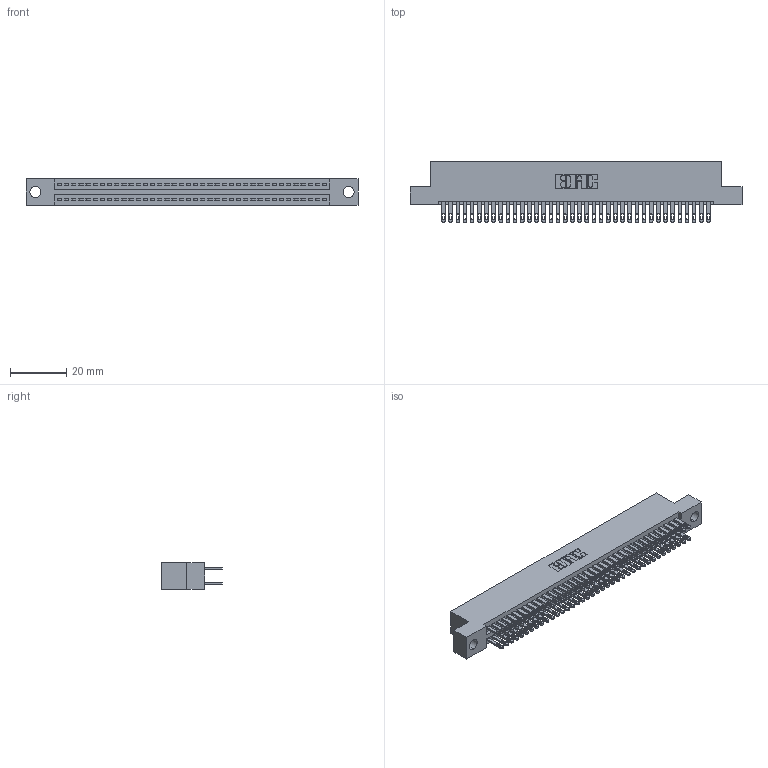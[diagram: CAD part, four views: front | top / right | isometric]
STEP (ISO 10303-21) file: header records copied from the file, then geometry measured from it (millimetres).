
FILE_DESCRIPTION (( 'STEP AP203' ), '1' );
FILE_NAME ('345-076-500-204.STEP', '2018-10-02T14:39:31', ( '' ), ( '' ), 'SwSTEP 2.0', 'SolidWorks 2016', '' );
FILE_SCHEMA (( 'CONFIG_CONTROL_DESIGN' ));
Length unit declared in the file: inch
Products named in the file (3): 345-292-001_345-293-100; 345-076-500-204; 345 Part_Flush Mounting Lugs - 0.156 Dia-TH
Assembly tree (77 placements, depth 2):
  345-076-500-204
    345 Part_Flush Mounting Lugs - 0.156 Dia-TH
    345-292-001_345-293-100  x76
Bounding box: 117.73 x 21.51 x 9.4 mm (x, y, z)
Volume: 11543.6 mm3; surface area: 17576.2 mm2
Topology: 77 solids, 77 shells, 3622 faces, 11057 edges, 7370 vertices
Faces by surface type: plane 2132, cylinder 1490
Entity records: 30287 total; most frequent: CARTESIAN_POINT 5080, ORIENTED_EDGE 5014, DIRECTION 4487, EDGE_CURVE 2507, VECTOR 2219, LINE 2219, VERTEX_POINT 1670, AXIS2_PLACEMENT_3D 1134
